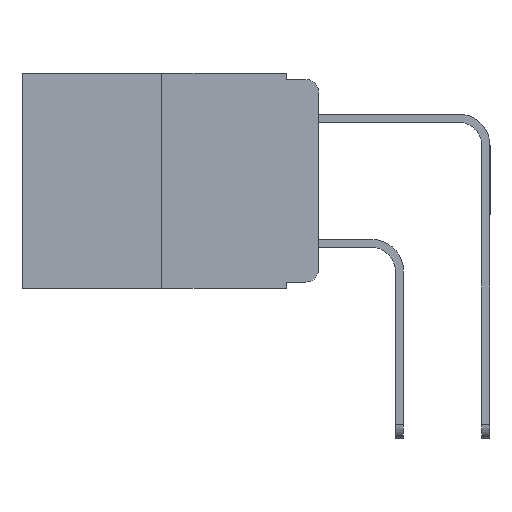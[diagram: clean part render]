
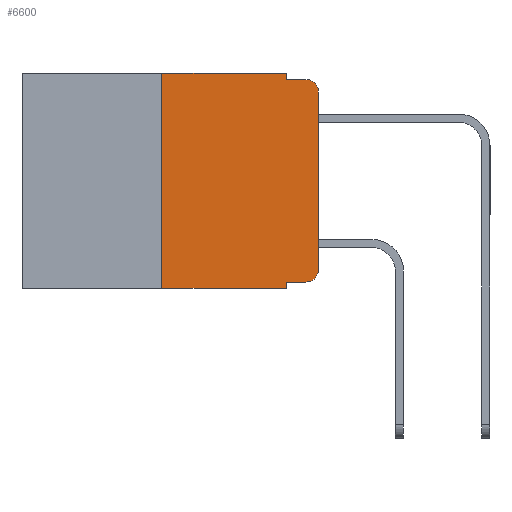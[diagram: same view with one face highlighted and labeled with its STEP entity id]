
A CAD part, left-side view. The second image highlights one B-rep face of the part: STEP entity #6600.
In plain terms, the highlighted planar face has unit normal (-1, 0, 0).
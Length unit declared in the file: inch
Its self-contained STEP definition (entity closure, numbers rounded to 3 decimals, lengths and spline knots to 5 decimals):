
#73 = CARTESIAN_POINT ( 'NONE',  ( 0., 0.473, -0.343 ) ) ;
#506 = DIRECTION ( 'NONE',  ( -1., 0., 0. ) ) ;
#793 = LINE ( 'NONE', #2796, #18432 ) ;
#807 = EDGE_CURVE ( 'NONE', #18132, #8446, #793, .T. ) ;
#945 = ORIENTED_EDGE ( 'NONE', *, *, #4193, .F. ) ;
#1334 = FACE_OUTER_BOUND ( 'NONE', #13145, .T. ) ;
#1936 = EDGE_CURVE ( 'NONE', #18132, #5987, #20560, .T. ) ;
#1990 = LINE ( 'NONE', #7441, #14467 ) ;
#2591 = VECTOR ( 'NONE', #8944, 39.37008 ) ;
#2743 = DIRECTION ( 'NONE',  ( 0., -1., 0. ) ) ;
#2796 = CARTESIAN_POINT ( 'NONE',  ( 0., 0.051, -0.333 ) ) ;
#3122 = LINE ( 'NONE', #73, #2591 ) ;
#3286 = CARTESIAN_POINT ( 'NONE',  ( 0., 0., -0.313 ) ) ;
#3845 = ORIENTED_EDGE ( 'NONE', *, *, #20163, .T. ) ;
#4193 = EDGE_CURVE ( 'NONE', #13173, #7969, #1990, .T. ) ;
#4284 = CARTESIAN_POINT ( 'NONE',  ( 0., 0.02, -0.333 ) ) ;
#4371 = ORIENTED_EDGE ( 'NONE', *, *, #6454, .F. ) ;
#4536 = CARTESIAN_POINT ( 'NONE',  ( 0., 0.051, -0.01 ) ) ;
#4718 = LINE ( 'NONE', #4536, #13338 ) ;
#5784 = CARTESIAN_POINT ( 'NONE',  ( 0., 0., 0. ) ) ;
#5813 = CARTESIAN_POINT ( 'NONE',  ( 0., 0.25, -0.343 ) ) ;
#5987 = VERTEX_POINT ( 'NONE', #8182 ) ;
#6454 = EDGE_CURVE ( 'NONE', #7633, #20318, #16309, .T. ) ;
#6481 = ORIENTED_EDGE ( 'NONE', *, *, #807, .T. ) ;
#6599 = CARTESIAN_POINT ( 'NONE',  ( 0., 0.02, -0.313 ) ) ;
#6600 = ADVANCED_FACE ( 'NONE', ( #1334 ), #14628, .F. ) ;
#6653 = EDGE_CURVE ( 'NONE', #7969, #7633, #17014, .T. ) ;
#7004 = ORIENTED_EDGE ( 'NONE', *, *, #10191, .T. ) ;
#7372 = DIRECTION ( 'NONE',  ( 0., 0., 1. ) ) ;
#7441 = CARTESIAN_POINT ( 'NONE',  ( 0., 0.25, 0. ) ) ;
#7569 = EDGE_CURVE ( 'NONE', #20318, #11058, #4718, .T. ) ;
#7633 = VERTEX_POINT ( 'NONE', #18546 ) ;
#7660 = CARTESIAN_POINT ( 'NONE',  ( 0., 0.051, -0.01 ) ) ;
#7969 = VERTEX_POINT ( 'NONE', #11612 ) ;
#8178 = VECTOR ( 'NONE', #20110, 39.37008 ) ;
#8182 = CARTESIAN_POINT ( 'NONE',  ( 0., 0.051, -0.343 ) ) ;
#8286 = DIRECTION ( 'NONE',  ( 0., 0., -1. ) ) ;
#8289 = EDGE_CURVE ( 'NONE', #12171, #11072, #17194, .T. ) ;
#8349 = CARTESIAN_POINT ( 'NONE',  ( 0., 0.051, 0. ) ) ;
#8372 = DIRECTION ( 'NONE',  ( 0., 0., -1. ) ) ;
#8446 = VERTEX_POINT ( 'NONE', #4284 ) ;
#8449 = VECTOR ( 'NONE', #10220, 39.37008 ) ;
#8625 = VECTOR ( 'NONE', #8372, 39.37008 ) ;
#8858 = EDGE_CURVE ( 'NONE', #13173, #5987, #3122, .T. ) ;
#8944 = DIRECTION ( 'NONE',  ( 0., -1., 0. ) ) ;
#9371 = DIRECTION ( 'NONE',  ( 1., 0., 0. ) ) ;
#10028 = AXIS2_PLACEMENT_3D ( 'NONE', #6599, #17673, #8286 ) ;
#10191 = EDGE_CURVE ( 'NONE', #8446, #12171, #14958, .T. ) ;
#10193 = CARTESIAN_POINT ( 'NONE',  ( 0., 0.051, 0. ) ) ;
#10220 = DIRECTION ( 'NONE',  ( 0., 0., -1. ) ) ;
#10510 = CARTESIAN_POINT ( 'NONE',  ( 0., 0.02, -0.03 ) ) ;
#10567 = CARTESIAN_POINT ( 'NONE',  ( 0., 0.02, -0.01 ) ) ;
#10633 = CARTESIAN_POINT ( 'NONE',  ( 0., 0., -0.03 ) ) ;
#10921 = CIRCLE ( 'NONE', #19716, 0.02 ) ;
#11058 = VERTEX_POINT ( 'NONE', #10567 ) ;
#11072 = VERTEX_POINT ( 'NONE', #10633 ) ;
#11612 = CARTESIAN_POINT ( 'NONE',  ( 0., 0.25, 0. ) ) ;
#11630 = CARTESIAN_POINT ( 'NONE',  ( 0., 0.473, 0. ) ) ;
#12038 = DIRECTION ( 'NONE',  ( 0., 0., -1. ) ) ;
#12078 = DIRECTION ( 'NONE',  ( 0., 0., -1. ) ) ;
#12171 = VERTEX_POINT ( 'NONE', #3286 ) ;
#12288 = AXIS2_PLACEMENT_3D ( 'NONE', #11630, #9371, #12038 ) ;
#12576 = VECTOR ( 'NONE', #13340, 39.37008 ) ;
#13014 = ORIENTED_EDGE ( 'NONE', *, *, #6653, .F. ) ;
#13145 = EDGE_LOOP ( 'NONE', ( #16196, #3845, #20752, #4371, #13014, #945, #13985, #18581, #6481, #7004 ) ) ;
#13173 = VERTEX_POINT ( 'NONE', #5813 ) ;
#13338 = VECTOR ( 'NONE', #13476, 39.37008 ) ;
#13340 = DIRECTION ( 'NONE',  ( 0., 0., 1. ) ) ;
#13476 = DIRECTION ( 'NONE',  ( 0., -1., 0. ) ) ;
#13985 = ORIENTED_EDGE ( 'NONE', *, *, #8858, .T. ) ;
#14467 = VECTOR ( 'NONE', #7372, 39.37008 ) ;
#14628 = PLANE ( 'NONE',  #12288 ) ;
#14958 = CIRCLE ( 'NONE', #10028, 0.02 ) ;
#16196 = ORIENTED_EDGE ( 'NONE', *, *, #8289, .T. ) ;
#16309 = LINE ( 'NONE', #10193, #8449 ) ;
#17014 = LINE ( 'NONE', #19093, #8178 ) ;
#17194 = LINE ( 'NONE', #5784, #12576 ) ;
#17673 = DIRECTION ( 'NONE',  ( -1., 0., 0. ) ) ;
#18132 = VERTEX_POINT ( 'NONE', #18784 ) ;
#18432 = VECTOR ( 'NONE', #2743, 39.37008 ) ;
#18546 = CARTESIAN_POINT ( 'NONE',  ( 0., 0.051, 0. ) ) ;
#18581 = ORIENTED_EDGE ( 'NONE', *, *, #1936, .F. ) ;
#18784 = CARTESIAN_POINT ( 'NONE',  ( 0., 0.051, -0.333 ) ) ;
#19093 = CARTESIAN_POINT ( 'NONE',  ( 0., 0.473, 0. ) ) ;
#19716 = AXIS2_PLACEMENT_3D ( 'NONE', #10510, #506, #12078 ) ;
#20110 = DIRECTION ( 'NONE',  ( 0., -1., 0. ) ) ;
#20163 = EDGE_CURVE ( 'NONE', #11072, #11058, #10921, .T. ) ;
#20318 = VERTEX_POINT ( 'NONE', #7660 ) ;
#20560 = LINE ( 'NONE', #8349, #8625 ) ;
#20752 = ORIENTED_EDGE ( 'NONE', *, *, #7569, .F. ) ;
